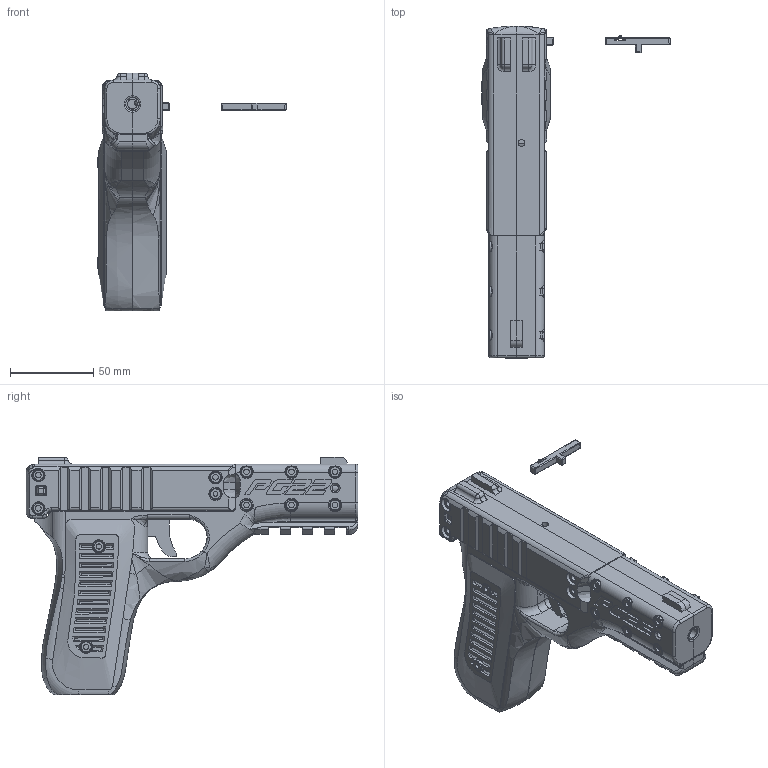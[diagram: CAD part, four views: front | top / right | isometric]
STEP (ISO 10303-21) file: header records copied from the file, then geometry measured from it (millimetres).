
FILE_DESCRIPTION(/* description */ (''),/* implementation_level */ '2;1');
FILE_NAME(/* name */ 'Aurora1.4.stp',/* time_stamp */ '2020-10-30T09:14:59-05:00',/* author */ (''),/* organization */ (''),/* preprocessor_version */ 'ST-DEVELOPER v15.2',/* originating_system */ 'Autodesk Translator Framework v2.0.0.5431',/* authorisation */ '');
FILE_SCHEMA (('AUTOMOTIVE_DESIGN { 1 0 10303 214 3 1 1 }'));
Products named in the file (1): Aurora1.4
Bounding box: 113.3 x 199.83 x 143.26 mm (x, y, z)
Volume: 381291.9 mm3; surface area: 152349.6 mm2
Topology: 47 solids, 47 shells, 1938 faces, 4808 edges, 3000 vertices
Faces by surface type: plane 935, cylinder 569, bspline 294, torus 109, sphere 16, cone 15
Full cylindrical faces by diameter (mm): 1.7 x1, 1.899 x1, 1.932 x1, 2.999 x1, 3.1 x1, 3.132 x4, 3.25 x3, 3.332 x14, 3.4 x1, 3.5 x1, 3.666 x24, 3.75 x3, 3.998 x18, 3.999 x4, 4.132 x4, 4.332 x19, 6 x1, 6.998 x18, 7.998 x11, 8 x1, 9.331 x1
Entity records: 69713 total; most frequent: CARTESIAN_POINT 25676, ORIENTED_EDGE 9164, DIRECTION 8541, EDGE_CURVE 4582, AXIS2_PLACEMENT_3D 2997, VERTEX_POINT 2985, LINE 2547, VECTOR 2547
